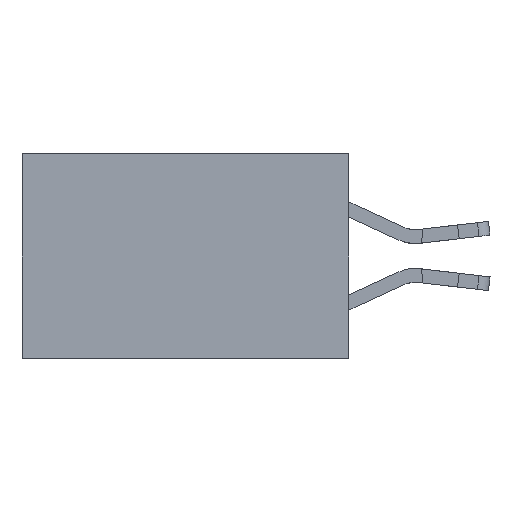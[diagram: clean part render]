
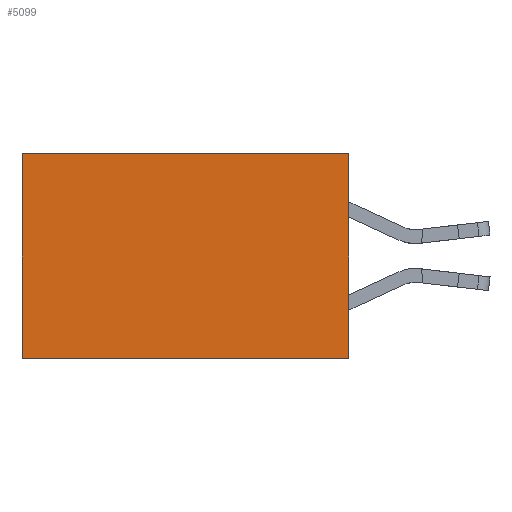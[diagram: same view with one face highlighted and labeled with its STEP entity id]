
A CAD part, left-side view. The second image highlights one B-rep face of the part: STEP entity #5099.
In plain terms, the highlighted planar face has unit normal (-1, 0, 0).
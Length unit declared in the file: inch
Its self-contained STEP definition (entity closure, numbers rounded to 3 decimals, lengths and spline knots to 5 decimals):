
#563 = FACE_OUTER_BOUND ( 'NONE', #686, .T. ) ;
#686 = EDGE_LOOP ( 'NONE', ( #11018, #28251, #10463, #21981 ) ) ;
#3158 = DIRECTION ( 'NONE',  ( 0., 1., 0. ) ) ;
#5099 = ADVANCED_FACE ( 'NONE', ( #563 ), #7076, .F. ) ;
#6425 = VECTOR ( 'NONE', #14710, 39.37008 ) ;
#6581 = EDGE_CURVE ( 'NONE', #18078, #19536, #27471, .T. ) ;
#6699 = VERTEX_POINT ( 'NONE', #21191 ) ;
#6964 = DIRECTION ( 'NONE',  ( 0., 0., -1. ) ) ;
#7033 = DIRECTION ( 'NONE',  ( 1., 0., 0. ) ) ;
#7076 = PLANE ( 'NONE',  #7507 ) ;
#7193 = LINE ( 'NONE', #21786, #6425 ) ;
#7507 = AXIS2_PLACEMENT_3D ( 'NONE', #8179, #7033, #6964 ) ;
#8179 = CARTESIAN_POINT ( 'NONE',  ( 0.277, 0., -0.37 ) ) ;
#9136 = CARTESIAN_POINT ( 'NONE',  ( 0.277, 0., 0. ) ) ;
#9844 = VECTOR ( 'NONE', #3158, 39.37008 ) ;
#10084 = VECTOR ( 'NONE', #17469, 39.37008 ) ;
#10463 = ORIENTED_EDGE ( 'NONE', *, *, #6581, .F. ) ;
#10826 = EDGE_CURVE ( 'NONE', #19536, #6699, #7193, .T. ) ;
#11018 = ORIENTED_EDGE ( 'NONE', *, *, #19731, .T. ) ;
#12480 = CARTESIAN_POINT ( 'NONE',  ( 0.277, 0.59, 0. ) ) ;
#14710 = DIRECTION ( 'NONE',  ( 0., 1., 0. ) ) ;
#16865 = CARTESIAN_POINT ( 'NONE',  ( 0.277, 0., -0.37 ) ) ;
#17469 = DIRECTION ( 'NONE',  ( 0., 0., -1. ) ) ;
#17731 = EDGE_CURVE ( 'NONE', #18078, #29840, #29375, .T. ) ;
#18078 = VERTEX_POINT ( 'NONE', #9136 ) ;
#19536 = VERTEX_POINT ( 'NONE', #16865 ) ;
#19731 = EDGE_CURVE ( 'NONE', #29840, #6699, #22693, .T. ) ;
#19776 = CARTESIAN_POINT ( 'NONE',  ( 0.277, 0., 0. ) ) ;
#21191 = CARTESIAN_POINT ( 'NONE',  ( 0.277, 0.59, -0.37 ) ) ;
#21786 = CARTESIAN_POINT ( 'NONE',  ( 0.277, 0., -0.37 ) ) ;
#21981 = ORIENTED_EDGE ( 'NONE', *, *, #17731, .T. ) ;
#22015 = VECTOR ( 'NONE', #23627, 39.37008 ) ;
#22693 = LINE ( 'NONE', #29151, #10084 ) ;
#23175 = CARTESIAN_POINT ( 'NONE',  ( 0.277, 0., -0.37 ) ) ;
#23627 = DIRECTION ( 'NONE',  ( 0., 0., -1. ) ) ;
#27471 = LINE ( 'NONE', #23175, #22015 ) ;
#28251 = ORIENTED_EDGE ( 'NONE', *, *, #10826, .F. ) ;
#29151 = CARTESIAN_POINT ( 'NONE',  ( 0.277, 0.59, -0.37 ) ) ;
#29375 = LINE ( 'NONE', #19776, #9844 ) ;
#29840 = VERTEX_POINT ( 'NONE', #12480 ) ;
